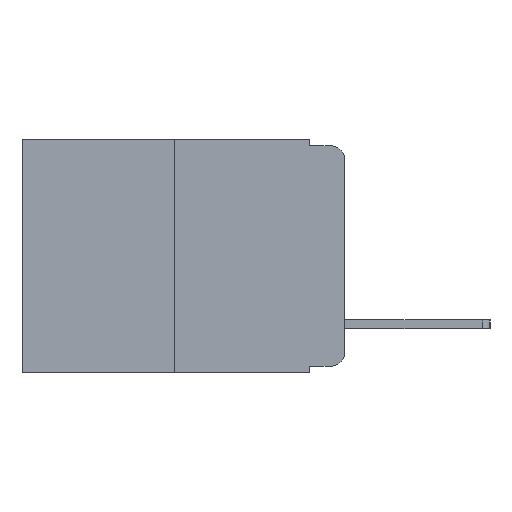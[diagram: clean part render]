
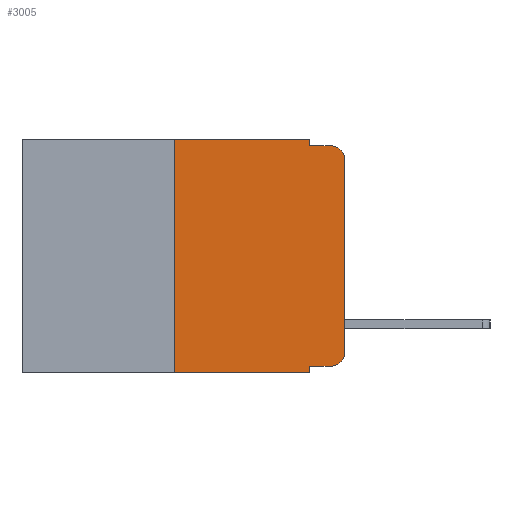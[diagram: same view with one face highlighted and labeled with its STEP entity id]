
A CAD part, left-side view. The second image highlights one B-rep face of the part: STEP entity #3005.
In plain terms, the highlighted planar face has unit normal (-1, 0, 0).
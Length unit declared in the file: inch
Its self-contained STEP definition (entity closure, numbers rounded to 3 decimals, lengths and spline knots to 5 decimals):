
#24 = DIRECTION ( 'NONE',  ( 0., -1., 0. ) ) ;
#153 = DIRECTION ( 'NONE',  ( -1., 0., 0. ) ) ;
#466 = VERTEX_POINT ( 'NONE', #3984 ) ;
#599 = ORIENTED_EDGE ( 'NONE', *, *, #14546, .T. ) ;
#907 = VERTEX_POINT ( 'NONE', #16295 ) ;
#968 = VERTEX_POINT ( 'NONE', #14524 ) ;
#1363 = AXIS2_PLACEMENT_3D ( 'NONE', #7068, #16023, #8394 ) ;
#1587 = EDGE_CURVE ( 'NONE', #3707, #466, #12896, .T. ) ;
#1711 = CARTESIAN_POINT ( 'NONE',  ( 0., 0.25, 0. ) ) ;
#2079 = VECTOR ( 'NONE', #11855, 39.37008 ) ;
#2156 = VERTEX_POINT ( 'NONE', #6094 ) ;
#2196 = ORIENTED_EDGE ( 'NONE', *, *, #4446, .T. ) ;
#2308 = VECTOR ( 'NONE', #12058, 39.37008 ) ;
#2715 = CARTESIAN_POINT ( 'NONE',  ( 0., 0.051, -0.01 ) ) ;
#2879 = ORIENTED_EDGE ( 'NONE', *, *, #1587, .F. ) ;
#3005 = ADVANCED_FACE ( 'NONE', ( #10226 ), #12259, .F. ) ;
#3039 = EDGE_CURVE ( 'NONE', #907, #2156, #16511, .T. ) ;
#3322 = LINE ( 'NONE', #1711, #16670 ) ;
#3535 = EDGE_CURVE ( 'NONE', #8471, #907, #3322, .T. ) ;
#3707 = VERTEX_POINT ( 'NONE', #5151 ) ;
#3984 = CARTESIAN_POINT ( 'NONE',  ( 0., 0.051, -0.343 ) ) ;
#4018 = ORIENTED_EDGE ( 'NONE', *, *, #3039, .F. ) ;
#4432 = ORIENTED_EDGE ( 'NONE', *, *, #13035, .T. ) ;
#4446 = EDGE_CURVE ( 'NONE', #12772, #6803, #7477, .T. ) ;
#4601 = LINE ( 'NONE', #13741, #14515 ) ;
#5151 = CARTESIAN_POINT ( 'NONE',  ( 0., 0.051, -0.333 ) ) ;
#5261 = VECTOR ( 'NONE', #8822, 39.37008 ) ;
#5402 = CIRCLE ( 'NONE', #1363, 0.02 ) ;
#5655 = ORIENTED_EDGE ( 'NONE', *, *, #8700, .T. ) ;
#5656 = EDGE_LOOP ( 'NONE', ( #7092, #2196, #13590, #6685, #4018, #14030, #5655, #2879, #599, #4432 ) ) ;
#5666 = LINE ( 'NONE', #10083, #5261 ) ;
#5737 = DIRECTION ( 'NONE',  ( 0., 0., -1. ) ) ;
#5759 = LINE ( 'NONE', #6600, #2079 ) ;
#5878 = EDGE_CURVE ( 'NONE', #16478, #12772, #4601, .T. ) ;
#6040 = CARTESIAN_POINT ( 'NONE',  ( 0., 0., -0.313 ) ) ;
#6094 = CARTESIAN_POINT ( 'NONE',  ( 0., 0.051, 0. ) ) ;
#6600 = CARTESIAN_POINT ( 'NONE',  ( 0., 0.051, -0.333 ) ) ;
#6685 = ORIENTED_EDGE ( 'NONE', *, *, #14447, .F. ) ;
#6803 = VERTEX_POINT ( 'NONE', #8772 ) ;
#6831 = AXIS2_PLACEMENT_3D ( 'NONE', #8453, #153, #9793 ) ;
#6999 = LINE ( 'NONE', #16698, #13492 ) ;
#7068 = CARTESIAN_POINT ( 'NONE',  ( 0., 0.02, -0.313 ) ) ;
#7092 = ORIENTED_EDGE ( 'NONE', *, *, #5878, .T. ) ;
#7115 = CARTESIAN_POINT ( 'NONE',  ( 0., 0.473, 0. ) ) ;
#7477 = CIRCLE ( 'NONE', #6831, 0.02 ) ;
#8054 = VERTEX_POINT ( 'NONE', #2715 ) ;
#8394 = DIRECTION ( 'NONE',  ( 0., 0., -1. ) ) ;
#8453 = CARTESIAN_POINT ( 'NONE',  ( 0., 0.02, -0.03 ) ) ;
#8471 = VERTEX_POINT ( 'NONE', #10479 ) ;
#8577 = AXIS2_PLACEMENT_3D ( 'NONE', #9669, #13534, #5737 ) ;
#8700 = EDGE_CURVE ( 'NONE', #8471, #466, #11685, .T. ) ;
#8772 = CARTESIAN_POINT ( 'NONE',  ( 0., 0.02, -0.01 ) ) ;
#8822 = DIRECTION ( 'NONE',  ( 0., -1., 0. ) ) ;
#9669 = CARTESIAN_POINT ( 'NONE',  ( 0., 0.473, 0. ) ) ;
#9682 = CARTESIAN_POINT ( 'NONE',  ( 0., 0.473, -0.343 ) ) ;
#9791 = DIRECTION ( 'NONE',  ( 0., -1., 0. ) ) ;
#9793 = DIRECTION ( 'NONE',  ( 0., 0., -1. ) ) ;
#10083 = CARTESIAN_POINT ( 'NONE',  ( 0., 0.051, -0.01 ) ) ;
#10226 = FACE_OUTER_BOUND ( 'NONE', #5656, .T. ) ;
#10479 = CARTESIAN_POINT ( 'NONE',  ( 0., 0.25, -0.343 ) ) ;
#10733 = EDGE_CURVE ( 'NONE', #8054, #6803, #5666, .T. ) ;
#11110 = DIRECTION ( 'NONE',  ( 0., 0., 1. ) ) ;
#11685 = LINE ( 'NONE', #9682, #16734 ) ;
#11755 = DIRECTION ( 'NONE',  ( 0., 0., -1. ) ) ;
#11855 = DIRECTION ( 'NONE',  ( 0., -1., 0. ) ) ;
#11872 = CARTESIAN_POINT ( 'NONE',  ( 0., 0., -0.03 ) ) ;
#12058 = DIRECTION ( 'NONE',  ( 0., 0., -1. ) ) ;
#12259 = PLANE ( 'NONE',  #8577 ) ;
#12772 = VERTEX_POINT ( 'NONE', #11872 ) ;
#12822 = VECTOR ( 'NONE', #9791, 39.37008 ) ;
#12896 = LINE ( 'NONE', #14564, #2308 ) ;
#13035 = EDGE_CURVE ( 'NONE', #968, #16478, #5402, .T. ) ;
#13492 = VECTOR ( 'NONE', #11755, 39.37008 ) ;
#13534 = DIRECTION ( 'NONE',  ( 1., 0., 0. ) ) ;
#13590 = ORIENTED_EDGE ( 'NONE', *, *, #10733, .F. ) ;
#13741 = CARTESIAN_POINT ( 'NONE',  ( 0., 0., 0. ) ) ;
#14030 = ORIENTED_EDGE ( 'NONE', *, *, #3535, .F. ) ;
#14447 = EDGE_CURVE ( 'NONE', #2156, #8054, #6999, .T. ) ;
#14515 = VECTOR ( 'NONE', #14992, 39.37008 ) ;
#14524 = CARTESIAN_POINT ( 'NONE',  ( 0., 0.02, -0.333 ) ) ;
#14546 = EDGE_CURVE ( 'NONE', #3707, #968, #5759, .T. ) ;
#14564 = CARTESIAN_POINT ( 'NONE',  ( 0., 0.051, 0. ) ) ;
#14992 = DIRECTION ( 'NONE',  ( 0., 0., 1. ) ) ;
#16023 = DIRECTION ( 'NONE',  ( -1., 0., 0. ) ) ;
#16295 = CARTESIAN_POINT ( 'NONE',  ( 0., 0.25, 0. ) ) ;
#16478 = VERTEX_POINT ( 'NONE', #6040 ) ;
#16511 = LINE ( 'NONE', #7115, #12822 ) ;
#16670 = VECTOR ( 'NONE', #11110, 39.37008 ) ;
#16698 = CARTESIAN_POINT ( 'NONE',  ( 0., 0.051, 0. ) ) ;
#16734 = VECTOR ( 'NONE', #24, 39.37008 ) ;
